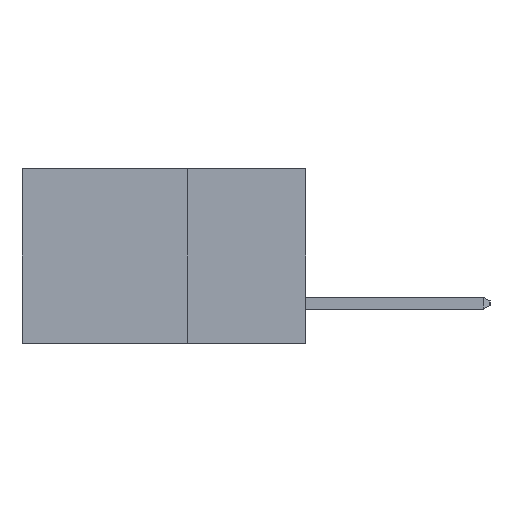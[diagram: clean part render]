
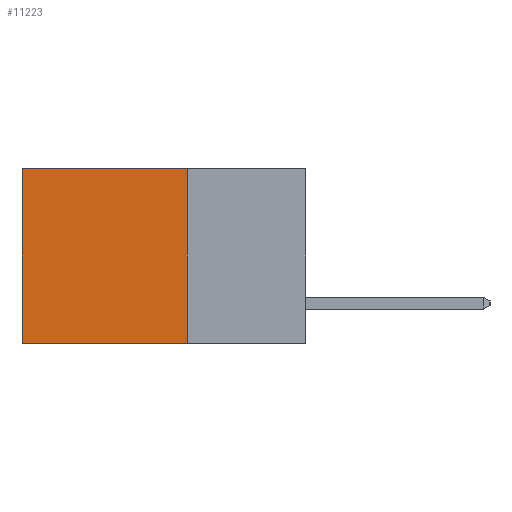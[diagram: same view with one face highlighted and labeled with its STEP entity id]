
A CAD part, left-side view. The second image highlights one B-rep face of the part: STEP entity #11223.
In plain terms, the highlighted planar face has unit normal (-1, 0, 0).
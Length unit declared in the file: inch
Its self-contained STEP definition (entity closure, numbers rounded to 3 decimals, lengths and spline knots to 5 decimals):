
#211 = CARTESIAN_POINT ( 'NONE',  ( 0.298, 0.25, -0.37 ) ) ;
#1076 = CARTESIAN_POINT ( 'NONE',  ( 0.298, 0.6, 0. ) ) ;
#1280 = ORIENTED_EDGE ( 'NONE', *, *, #13262, .F. ) ;
#1687 = CARTESIAN_POINT ( 'NONE',  ( 0.298, 0.25, 0. ) ) ;
#1761 = EDGE_CURVE ( 'NONE', #11649, #10109, #4361, .T. ) ;
#2126 = CARTESIAN_POINT ( 'NONE',  ( 0.298, 0.6, -0.37 ) ) ;
#2345 = VECTOR ( 'NONE', #6129, 39.37008 ) ;
#2670 = EDGE_LOOP ( 'NONE', ( #12972, #3775, #1280, #7972 ) ) ;
#3708 = CARTESIAN_POINT ( 'NONE',  ( 0.298, 0.25, -0.37 ) ) ;
#3775 = ORIENTED_EDGE ( 'NONE', *, *, #7638, .F. ) ;
#4361 = LINE ( 'NONE', #1076, #7120 ) ;
#4380 = CARTESIAN_POINT ( 'NONE',  ( 0.298, 0.6, 0. ) ) ;
#4528 = FACE_OUTER_BOUND ( 'NONE', #2670, .T. ) ;
#4742 = DIRECTION ( 'NONE',  ( 1., 0., 0. ) ) ;
#5073 = CARTESIAN_POINT ( 'NONE',  ( 0.298, 0.25, 0. ) ) ;
#5594 = AXIS2_PLACEMENT_3D ( 'NONE', #9874, #4742, #11966 ) ;
#6129 = DIRECTION ( 'NONE',  ( 0., 0., -1. ) ) ;
#6745 = LINE ( 'NONE', #211, #11877 ) ;
#7120 = VECTOR ( 'NONE', #13153, 39.37008 ) ;
#7638 = EDGE_CURVE ( 'NONE', #11751, #10109, #6745, .T. ) ;
#7805 = VERTEX_POINT ( 'NONE', #9891 ) ;
#7852 = EDGE_CURVE ( 'NONE', #7805, #11649, #9286, .T. ) ;
#7972 = ORIENTED_EDGE ( 'NONE', *, *, #7852, .T. ) ;
#8921 = DIRECTION ( 'NONE',  ( 0., 1., 0. ) ) ;
#9286 = LINE ( 'NONE', #1687, #9610 ) ;
#9610 = VECTOR ( 'NONE', #8921, 39.37008 ) ;
#9874 = CARTESIAN_POINT ( 'NONE',  ( 0.298, 0.25, 0. ) ) ;
#9891 = CARTESIAN_POINT ( 'NONE',  ( 0.298, 0.25, 0. ) ) ;
#10109 = VERTEX_POINT ( 'NONE', #2126 ) ;
#10276 = LINE ( 'NONE', #5073, #2345 ) ;
#10605 = DIRECTION ( 'NONE',  ( 0., 1., 0. ) ) ;
#10906 = PLANE ( 'NONE',  #5594 ) ;
#11223 = ADVANCED_FACE ( 'NONE', ( #4528 ), #10906, .F. ) ;
#11649 = VERTEX_POINT ( 'NONE', #4380 ) ;
#11751 = VERTEX_POINT ( 'NONE', #3708 ) ;
#11877 = VECTOR ( 'NONE', #10605, 39.37008 ) ;
#11966 = DIRECTION ( 'NONE',  ( 0., 0., -1. ) ) ;
#12972 = ORIENTED_EDGE ( 'NONE', *, *, #1761, .T. ) ;
#13153 = DIRECTION ( 'NONE',  ( 0., 0., -1. ) ) ;
#13262 = EDGE_CURVE ( 'NONE', #7805, #11751, #10276, .T. ) ;
